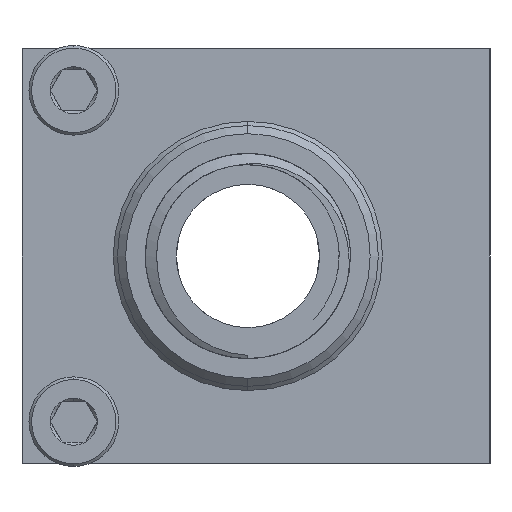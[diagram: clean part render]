
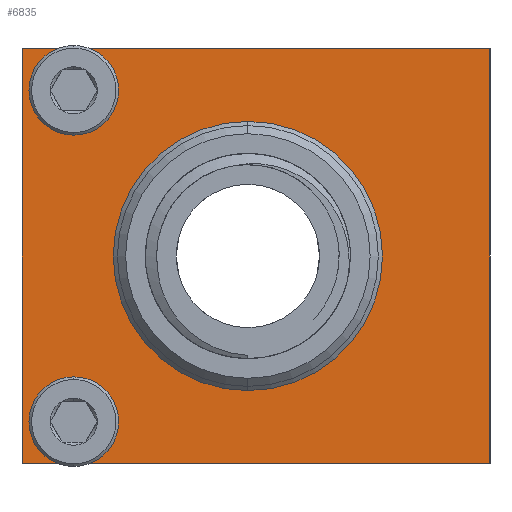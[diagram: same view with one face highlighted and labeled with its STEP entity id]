
A CAD part, left-side view. The second image highlights one B-rep face of the part: STEP entity #6835.
In plain terms, the highlighted face is planar.
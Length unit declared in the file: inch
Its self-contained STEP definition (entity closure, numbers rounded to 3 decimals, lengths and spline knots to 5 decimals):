
#126 = ORIENTED_EDGE ( 'NONE', *, *, #12727, .T. ) ;
#1342 = DIRECTION ( 'NONE',  ( 1., 0., 0. ) ) ;
#1547 = CARTESIAN_POINT ( 'NONE',  ( 1., 0., 0. ) ) ;
#1966 = LINE ( 'NONE', #18236, #7054 ) ;
#2492 = DIRECTION ( 'NONE',  ( 1., 0., 0. ) ) ;
#2596 = VERTEX_POINT ( 'NONE', #19049 ) ;
#2798 = CIRCLE ( 'NONE', #12406, 0.06693 ) ;
#2905 = CARTESIAN_POINT ( 'NONE',  ( 0.16693, -0.125, 0. ) ) ;
#2930 = AXIS2_PLACEMENT_3D ( 'NONE', #17255, #22579, #9902 ) ;
#2979 = EDGE_CURVE ( 'NONE', #6038, #8442, #17681, .T. ) ;
#3487 = FACE_BOUND ( 'NONE', #22723, .T. ) ;
#3605 = DIRECTION ( 'NONE',  ( 1., 0., 0. ) ) ;
#3880 = VERTEX_POINT ( 'NONE', #19302 ) ;
#4003 = EDGE_LOOP ( 'NONE', ( #17375, #17446 ) ) ;
#4098 = EDGE_CURVE ( 'NONE', #3880, #13582, #8471, .T. ) ;
#4239 = AXIS2_PLACEMENT_3D ( 'NONE', #4832, #12207, #17725 ) ;
#4615 = EDGE_LOOP ( 'NONE', ( #17954, #5754, #8127, #9110 ) ) ;
#4620 = DIRECTION ( 'NONE',  ( 0., 0., 1. ) ) ;
#4736 = DIRECTION ( 'NONE',  ( -1., 0., 0. ) ) ;
#4832 = CARTESIAN_POINT ( 'NONE',  ( 0.9, -0.125, 0. ) ) ;
#5277 = FACE_BOUND ( 'NONE', #4003, .T. ) ;
#5398 = PLANE ( 'NONE',  #18957 ) ;
#5576 = CIRCLE ( 'NONE', #20606, 0.325 ) ;
#5655 = ORIENTED_EDGE ( 'NONE', *, *, #2979, .T. ) ;
#5754 = ORIENTED_EDGE ( 'NONE', *, *, #14458, .F. ) ;
#5868 = VERTEX_POINT ( 'NONE', #12119 ) ;
#6038 = VERTEX_POINT ( 'NONE', #6419 ) ;
#6086 = EDGE_CURVE ( 'NONE', #13582, #3880, #2798, .T. ) ;
#6384 = CIRCLE ( 'NONE', #2930, 0.06693 ) ;
#6419 = CARTESIAN_POINT ( 'NONE',  ( 0.03307, -0.125, 0. ) ) ;
#6835 = ADVANCED_FACE ( 'NONE', ( #7100, #5277, #3487, #7222 ), #5398, .F. ) ;
#6985 = CARTESIAN_POINT ( 'NONE',  ( 0.5, -0.5454, 0. ) ) ;
#7054 = VECTOR ( 'NONE', #11377, 39.37008 ) ;
#7086 = EDGE_CURVE ( 'NONE', #15689, #9620, #1966, .T. ) ;
#7100 = FACE_BOUND ( 'NONE', #11357, .T. ) ;
#7222 = FACE_OUTER_BOUND ( 'NONE', #4615, .T. ) ;
#7432 = VERTEX_POINT ( 'NONE', #15951 ) ;
#8127 = ORIENTED_EDGE ( 'NONE', *, *, #16162, .F. ) ;
#8442 = VERTEX_POINT ( 'NONE', #2905 ) ;
#8471 = CIRCLE ( 'NONE', #4239, 0.06693 ) ;
#9110 = ORIENTED_EDGE ( 'NONE', *, *, #9199, .F. ) ;
#9199 = EDGE_CURVE ( 'NONE', #9620, #2596, #14485, .T. ) ;
#9253 = DIRECTION ( 'NONE',  ( 0., 1., 0. ) ) ;
#9620 = VERTEX_POINT ( 'NONE', #10189 ) ;
#9902 = DIRECTION ( 'NONE',  ( 1., 0., 0. ) ) ;
#9983 = CIRCLE ( 'NONE', #15391, 0.325 ) ;
#10189 = CARTESIAN_POINT ( 'NONE',  ( 0., -1.13, 0. ) ) ;
#10709 = DIRECTION ( 'NONE',  ( 1., 0., 0. ) ) ;
#11357 = EDGE_LOOP ( 'NONE', ( #13394, #5655 ) ) ;
#11377 = DIRECTION ( 'NONE',  ( 0., -1., 0. ) ) ;
#11564 = VERTEX_POINT ( 'NONE', #16535 ) ;
#11718 = CARTESIAN_POINT ( 'NONE',  ( 0.96693, -0.125, 0. ) ) ;
#12119 = CARTESIAN_POINT ( 'NONE',  ( 1., 0., 0. ) ) ;
#12137 = DIRECTION ( 'NONE',  ( 0., 0., 1. ) ) ;
#12207 = DIRECTION ( 'NONE',  ( 0., 0., 1. ) ) ;
#12406 = AXIS2_PLACEMENT_3D ( 'NONE', #15831, #14240, #1342 ) ;
#12727 = EDGE_CURVE ( 'NONE', #7432, #11564, #9983, .T. ) ;
#12766 = CARTESIAN_POINT ( 'NONE',  ( 0., 0., 0. ) ) ;
#13394 = ORIENTED_EDGE ( 'NONE', *, *, #20207, .T. ) ;
#13430 = CARTESIAN_POINT ( 'NONE',  ( 0.1, -0.125, 0. ) ) ;
#13444 = CARTESIAN_POINT ( 'NONE',  ( 0., 0., 0. ) ) ;
#13582 = VERTEX_POINT ( 'NONE', #11718 ) ;
#14240 = DIRECTION ( 'NONE',  ( 0., 0., 1. ) ) ;
#14449 = DIRECTION ( 'NONE',  ( 0., 0., 1. ) ) ;
#14458 = EDGE_CURVE ( 'NONE', #5868, #15689, #15612, .T. ) ;
#14485 = LINE ( 'NONE', #19657, #22918 ) ;
#14807 = VECTOR ( 'NONE', #4736, 39.37008 ) ;
#15243 = ORIENTED_EDGE ( 'NONE', *, *, #19601, .T. ) ;
#15391 = AXIS2_PLACEMENT_3D ( 'NONE', #6985, #14449, #10709 ) ;
#15612 = LINE ( 'NONE', #17754, #14807 ) ;
#15689 = VERTEX_POINT ( 'NONE', #13444 ) ;
#15831 = CARTESIAN_POINT ( 'NONE',  ( 0.9, -0.125, 0. ) ) ;
#15951 = CARTESIAN_POINT ( 'NONE',  ( 0.825, -0.5454, 0. ) ) ;
#16162 = EDGE_CURVE ( 'NONE', #2596, #5868, #18046, .T. ) ;
#16535 = CARTESIAN_POINT ( 'NONE',  ( 0.175, -0.5454, 0. ) ) ;
#17255 = CARTESIAN_POINT ( 'NONE',  ( 0.1, -0.125, 0. ) ) ;
#17375 = ORIENTED_EDGE ( 'NONE', *, *, #6086, .T. ) ;
#17446 = ORIENTED_EDGE ( 'NONE', *, *, #4098, .T. ) ;
#17681 = CIRCLE ( 'NONE', #20786, 0.06693 ) ;
#17725 = DIRECTION ( 'NONE',  ( 1., 0., 0. ) ) ;
#17754 = CARTESIAN_POINT ( 'NONE',  ( 0., 0., 0. ) ) ;
#17954 = ORIENTED_EDGE ( 'NONE', *, *, #7086, .F. ) ;
#18046 = LINE ( 'NONE', #1547, #19857 ) ;
#18088 = DIRECTION ( 'NONE',  ( 1., 0., 0. ) ) ;
#18236 = CARTESIAN_POINT ( 'NONE',  ( 0., 0., 0. ) ) ;
#18957 = AXIS2_PLACEMENT_3D ( 'NONE', #12766, #20104, #3605 ) ;
#18965 = DIRECTION ( 'NONE',  ( 1., 0., 0. ) ) ;
#19049 = CARTESIAN_POINT ( 'NONE',  ( 1., -1.13, 0. ) ) ;
#19302 = CARTESIAN_POINT ( 'NONE',  ( 0.83307, -0.125, 0. ) ) ;
#19601 = EDGE_CURVE ( 'NONE', #11564, #7432, #5576, .T. ) ;
#19657 = CARTESIAN_POINT ( 'NONE',  ( 0., -1.13, 0. ) ) ;
#19857 = VECTOR ( 'NONE', #9253, 39.37008 ) ;
#20104 = DIRECTION ( 'NONE',  ( 0., 0., 1. ) ) ;
#20207 = EDGE_CURVE ( 'NONE', #8442, #6038, #6384, .T. ) ;
#20606 = AXIS2_PLACEMENT_3D ( 'NONE', #21409, #12137, #2492 ) ;
#20786 = AXIS2_PLACEMENT_3D ( 'NONE', #13430, #4620, #18965 ) ;
#21409 = CARTESIAN_POINT ( 'NONE',  ( 0.5, -0.5454, 0. ) ) ;
#22579 = DIRECTION ( 'NONE',  ( 0., 0., 1. ) ) ;
#22723 = EDGE_LOOP ( 'NONE', ( #126, #15243 ) ) ;
#22918 = VECTOR ( 'NONE', #18088, 39.37008 ) ;
